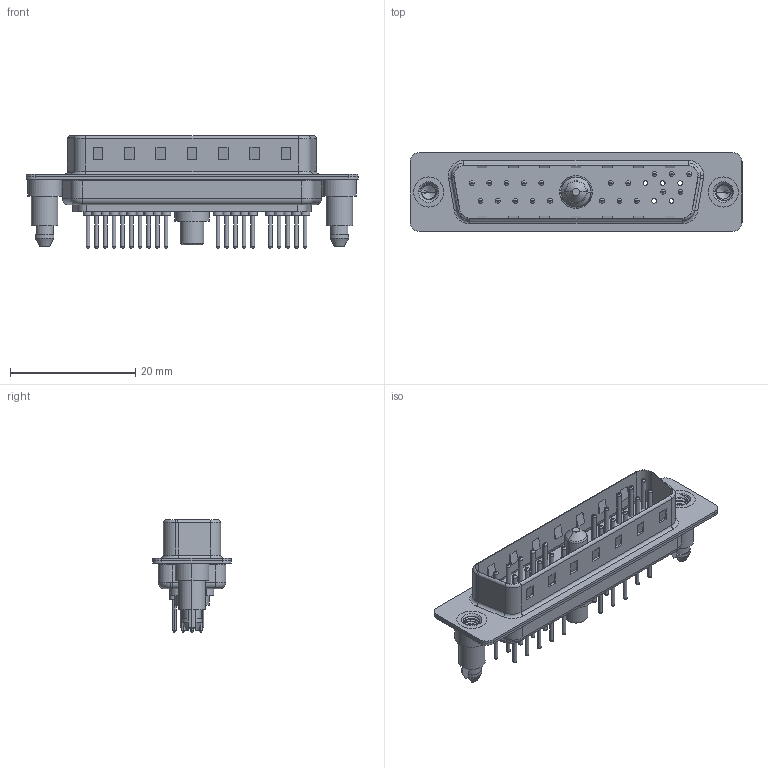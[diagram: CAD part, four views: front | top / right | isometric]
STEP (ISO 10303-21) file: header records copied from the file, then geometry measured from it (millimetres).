
FILE_DESCRIPTION (( 'STEP AP203' ), '1' );
FILE_NAME ('627-21W1224-4ND.STEP', '2019-05-28T00:30:30', ( '' ), ( '' ), 'SwSTEP 2.0', 'SolidWorks 2016', '' );
FILE_SCHEMA (( 'CONFIG_CONTROL_DESIGN' ));
Length unit declared in the file: millimetre
Products named in the file (9): 627Combo Contact Row 2_24; 627-21W1224-4ND; 627Combo Shell Front_25 Contacts; Power Pin_40A S; 627Combo Threaded Boardlock_D; 627Combo Threaded Boardlock_5; 627Combo Contact Row 1_24; 627Combo Shell Rear_25 Contacts; 627Combo Housing_21W1
Assembly tree (26 placements, depth 2):
  627-21W1224-4ND
    627Combo Housing_21W1
    627Combo Shell Rear_25 Contacts
    627Combo Shell Front_25 Contacts
    627Combo Threaded Boardlock_D
    Power Pin_40A S
    627Combo Threaded Boardlock_5
    627Combo Contact Row 1_24  x10
    627Combo Contact Row 2_24  x10
Bounding box: 53 x 12.6 x 17.9 mm (x, y, z)
Volume: 2940.5 mm3; surface area: 7174.7 mm2
Topology: 27 solids, 27 shells, 1214 faces, 2674 edges, 1632 vertices
Faces by surface type: cylinder 476, torus 372, plane 337, cone 20, bspline 9
Entity records: 25555 total; most frequent: CARTESIAN_POINT 7522, DIRECTION 3668, ORIENTED_EDGE 3320, EDGE_CURVE 1660, AXIS2_PLACEMENT_3D 1437, VERTEX_POINT 1056, EDGE_LOOP 844, VECTOR 794
